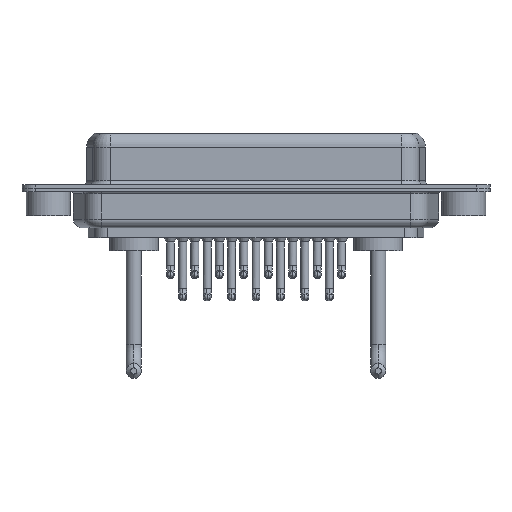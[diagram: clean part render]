
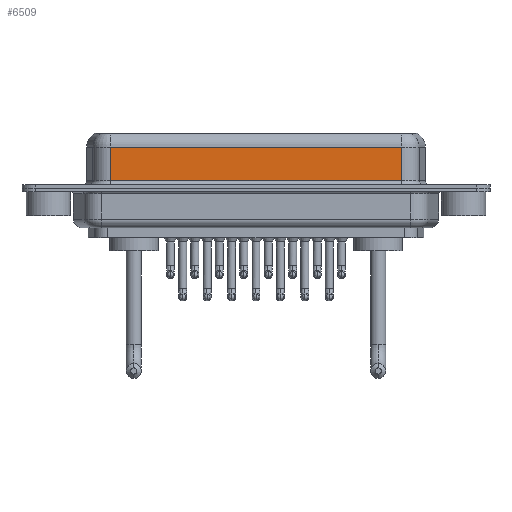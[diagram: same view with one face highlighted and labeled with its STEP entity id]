
A CAD part, front view. The second image highlights one B-rep face of the part: STEP entity #6509.
In plain terms, the highlighted planar face has unit normal (0, -1, 0).
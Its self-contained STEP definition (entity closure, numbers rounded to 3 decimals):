
#495 = EDGE_CURVE ( 'NONE', #19112, #20881, #13462, .T. ) ;
#527 = CARTESIAN_POINT ( 'NONE',  ( 7.013, -3.95, 6.4 ) ) ;
#1415 = ORIENTED_EDGE ( 'NONE', *, *, #4414, .T. ) ;
#2884 = AXIS2_PLACEMENT_3D ( 'NONE', #13571, #20004, #3156 ) ;
#3156 = DIRECTION ( 'NONE',  ( 0., 0., 1. ) ) ;
#3600 = DIRECTION ( 'NONE',  ( 0., 0., -1. ) ) ;
#3978 = VERTEX_POINT ( 'NONE', #12603 ) ;
#4414 = EDGE_CURVE ( 'NONE', #19112, #16823, #10567, .T. ) ;
#6509 = ADVANCED_FACE ( 'NONE', ( #13874 ), #20313, .F. ) ;
#6653 = VECTOR ( 'NONE', #3600, 1000. ) ;
#6658 = LINE ( 'NONE', #527, #6653 ) ;
#6923 = ORIENTED_EDGE ( 'NONE', *, *, #9570, .T. ) ;
#6996 = CARTESIAN_POINT ( 'NONE',  ( 7.013, -3.95, 4.65 ) ) ;
#8108 = EDGE_LOOP ( 'NONE', ( #17523, #1415, #6923, #19375 ) ) ;
#9570 = EDGE_CURVE ( 'NONE', #16823, #3978, #6658, .T. ) ;
#10025 = CARTESIAN_POINT ( 'NONE',  ( 40.037, -3.95, 0.9 ) ) ;
#10383 = CARTESIAN_POINT ( 'NONE',  ( 40.037, -3.95, 6.4 ) ) ;
#10567 = LINE ( 'NONE', #11959, #15981 ) ;
#11031 = LINE ( 'NONE', #17046, #12916 ) ;
#11959 = CARTESIAN_POINT ( 'NONE',  ( 40.037, -3.95, 4.65 ) ) ;
#12603 = CARTESIAN_POINT ( 'NONE',  ( 7.013, -3.95, 0.9 ) ) ;
#12916 = VECTOR ( 'NONE', #20636, 1000. ) ;
#13462 = LINE ( 'NONE', #10383, #15920 ) ;
#13571 = CARTESIAN_POINT ( 'NONE',  ( 40.037, -3.95, 6.4 ) ) ;
#13874 = FACE_OUTER_BOUND ( 'NONE', #8108, .T. ) ;
#14934 = DIRECTION ( 'NONE',  ( 0., 0., -1. ) ) ;
#15920 = VECTOR ( 'NONE', #14934, 1000. ) ;
#15981 = VECTOR ( 'NONE', #16999, 1000. ) ;
#16823 = VERTEX_POINT ( 'NONE', #6996 ) ;
#16999 = DIRECTION ( 'NONE',  ( -1., 0., 0. ) ) ;
#17046 = CARTESIAN_POINT ( 'NONE',  ( 40.037, -3.95, 0.9 ) ) ;
#17402 = CARTESIAN_POINT ( 'NONE',  ( 40.037, -3.95, 4.65 ) ) ;
#17523 = ORIENTED_EDGE ( 'NONE', *, *, #495, .F. ) ;
#19112 = VERTEX_POINT ( 'NONE', #17402 ) ;
#19375 = ORIENTED_EDGE ( 'NONE', *, *, #19641, .T. ) ;
#19641 = EDGE_CURVE ( 'NONE', #3978, #20881, #11031, .T. ) ;
#20004 = DIRECTION ( 'NONE',  ( 0., 1., 0. ) ) ;
#20313 = PLANE ( 'NONE',  #2884 ) ;
#20636 = DIRECTION ( 'NONE',  ( 1., 0., 0. ) ) ;
#20881 = VERTEX_POINT ( 'NONE', #10025 ) ;
